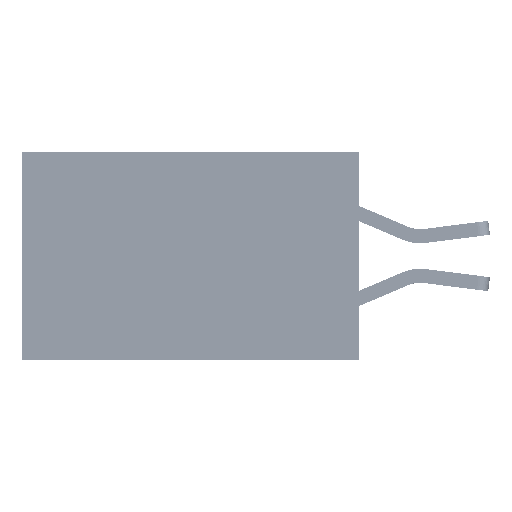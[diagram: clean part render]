
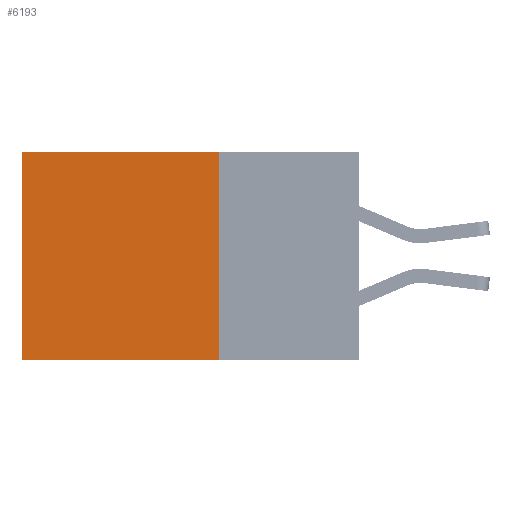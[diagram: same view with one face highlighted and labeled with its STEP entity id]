
A CAD part, left-side view. The second image highlights one B-rep face of the part: STEP entity #6193.
In plain terms, the highlighted planar face has unit normal (-1, 0, 0).
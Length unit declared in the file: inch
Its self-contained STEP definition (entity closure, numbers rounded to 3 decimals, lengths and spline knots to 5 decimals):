
#738 = CARTESIAN_POINT ( 'NONE',  ( 0.2875, 0.6, 0. ) ) ;
#2273 = VERTEX_POINT ( 'NONE', #9497 ) ;
#4398 = VERTEX_POINT ( 'NONE', #6618 ) ;
#4657 = AXIS2_PLACEMENT_3D ( 'NONE', #5791, #17204, #28310 ) ;
#5791 = CARTESIAN_POINT ( 'NONE',  ( 0.2875, 0.25, 0. ) ) ;
#6193 = ADVANCED_FACE ( 'NONE', ( #38276 ), #38298, .F. ) ;
#6618 = CARTESIAN_POINT ( 'NONE',  ( 0.2875, 0.6, -0.37 ) ) ;
#8619 = VECTOR ( 'NONE', #24165, 39.37008 ) ;
#9293 = CARTESIAN_POINT ( 'NONE',  ( 0.2875, 0.25, 0. ) ) ;
#9497 = CARTESIAN_POINT ( 'NONE',  ( 0.2875, 0.25, -0.37 ) ) ;
#11635 = VERTEX_POINT ( 'NONE', #738 ) ;
#12350 = VECTOR ( 'NONE', #35673, 39.37008 ) ;
#14118 = VECTOR ( 'NONE', #32269, 39.37008 ) ;
#15283 = EDGE_CURVE ( 'NONE', #25439, #11635, #25669, .T. ) ;
#16899 = LINE ( 'NONE', #28062, #14118 ) ;
#17204 = DIRECTION ( 'NONE',  ( 1., 0., 0. ) ) ;
#18285 = EDGE_CURVE ( 'NONE', #25439, #2273, #25986, .T. ) ;
#18575 = EDGE_LOOP ( 'NONE', ( #40865, #25727, #19247, #20034 ) ) ;
#19247 = ORIENTED_EDGE ( 'NONE', *, *, #18285, .F. ) ;
#19703 = EDGE_CURVE ( 'NONE', #11635, #4398, #16899, .T. ) ;
#20034 = ORIENTED_EDGE ( 'NONE', *, *, #15283, .T. ) ;
#24165 = DIRECTION ( 'NONE',  ( 0., 0., -1. ) ) ;
#25439 = VERTEX_POINT ( 'NONE', #25917 ) ;
#25669 = LINE ( 'NONE', #42247, #28490 ) ;
#25727 = ORIENTED_EDGE ( 'NONE', *, *, #28909, .F. ) ;
#25917 = CARTESIAN_POINT ( 'NONE',  ( 0.2875, 0.25, 0. ) ) ;
#25986 = LINE ( 'NONE', #9293, #8619 ) ;
#28062 = CARTESIAN_POINT ( 'NONE',  ( 0.2875, 0.6, 0. ) ) ;
#28310 = DIRECTION ( 'NONE',  ( 0., 0., -1. ) ) ;
#28490 = VECTOR ( 'NONE', #38344, 39.37008 ) ;
#28569 = LINE ( 'NONE', #32249, #12350 ) ;
#28909 = EDGE_CURVE ( 'NONE', #2273, #4398, #28569, .T. ) ;
#32249 = CARTESIAN_POINT ( 'NONE',  ( 0.2875, 0.25, -0.37 ) ) ;
#32269 = DIRECTION ( 'NONE',  ( 0., 0., -1. ) ) ;
#35673 = DIRECTION ( 'NONE',  ( 0., 1., 0. ) ) ;
#38276 = FACE_OUTER_BOUND ( 'NONE', #18575, .T. ) ;
#38298 = PLANE ( 'NONE',  #4657 ) ;
#38344 = DIRECTION ( 'NONE',  ( 0., 1., 0. ) ) ;
#40865 = ORIENTED_EDGE ( 'NONE', *, *, #19703, .T. ) ;
#42247 = CARTESIAN_POINT ( 'NONE',  ( 0.2875, 0.25, 0. ) ) ;
